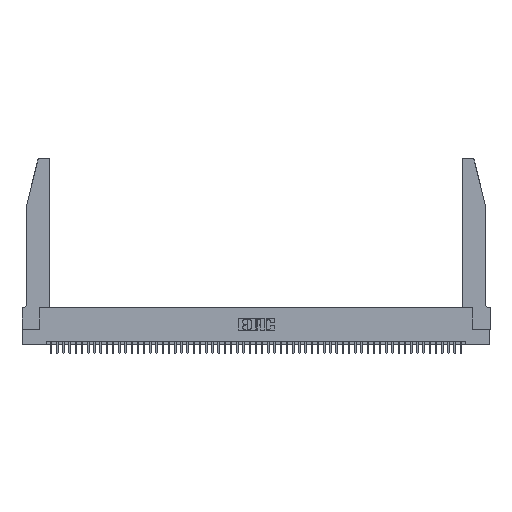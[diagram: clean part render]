
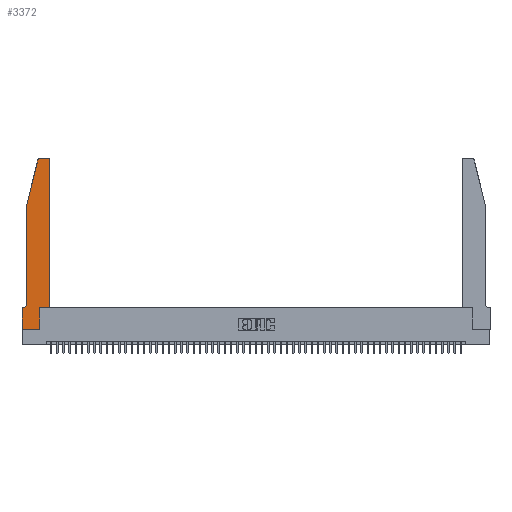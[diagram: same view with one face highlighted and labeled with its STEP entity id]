
A CAD part, top view. The second image highlights one B-rep face of the part: STEP entity #3372.
In plain terms, the highlighted planar face has unit normal (0, 0, 1).
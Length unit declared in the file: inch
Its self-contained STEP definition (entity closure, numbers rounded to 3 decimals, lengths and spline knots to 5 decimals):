
#15 = EDGE_CURVE ( 'NONE', #44403, #13688, #19117, .T. ) ;
#131 = VECTOR ( 'NONE', #29514, 39.37008 ) ;
#475 = ORIENTED_EDGE ( 'NONE', *, *, #31241, .T. ) ;
#2069 = CARTESIAN_POINT ( 'NONE',  ( 0.0755, 2., 0.37 ) ) ;
#2253 = CARTESIAN_POINT ( 'NONE',  ( 0.0755, 0.35, 0.37 ) ) ;
#2636 = CIRCLE ( 'NONE', #48445, 0.03 ) ;
#3372 = ADVANCED_FACE ( 'NONE', ( #43857 ), #22199, .T. ) ;
#3374 = CARTESIAN_POINT ( 'NONE',  ( 0., 0.35, 0.37 ) ) ;
#3427 = VECTOR ( 'NONE', #8795, 39.37008 ) ;
#3840 = LINE ( 'NONE', #7903, #22732 ) ;
#4207 = CARTESIAN_POINT ( 'NONE',  ( 0.284, 2.75, 0.37 ) ) ;
#5001 = CARTESIAN_POINT ( 'NONE',  ( 0.2865, 0.35, 0.37 ) ) ;
#5003 = DIRECTION ( 'NONE',  ( -1., 0., 0. ) ) ;
#5638 = CARTESIAN_POINT ( 'NONE',  ( 0., 0., 0.37 ) ) ;
#6125 = VERTEX_POINT ( 'NONE', #37381 ) ;
#6273 = DIRECTION ( 'NONE',  ( 0., 0., -1. ) ) ;
#7343 = CARTESIAN_POINT ( 'NONE',  ( 0.0055, 0.35, 0.37 ) ) ;
#7903 = CARTESIAN_POINT ( 'NONE',  ( 0., 0., 0.37 ) ) ;
#8156 = LINE ( 'NONE', #51438, #11471 ) ;
#8225 = AXIS2_PLACEMENT_3D ( 'NONE', #10287, #6273, #47514 ) ;
#8795 = DIRECTION ( 'NONE',  ( 0., 1., 0. ) ) ;
#8818 = VECTOR ( 'NONE', #5003, 39.37008 ) ;
#9454 = LINE ( 'NONE', #33608, #8818 ) ;
#9557 = ORIENTED_EDGE ( 'NONE', *, *, #22637, .T. ) ;
#10287 = CARTESIAN_POINT ( 'NONE',  ( 0.0055, 0.42, 0.37 ) ) ;
#10353 = ORIENTED_EDGE ( 'NONE', *, *, #49988, .T. ) ;
#11436 = VERTEX_POINT ( 'NONE', #46766 ) ;
#11471 = VECTOR ( 'NONE', #38810, 39.37008 ) ;
#12121 = CARTESIAN_POINT ( 'NONE',  ( 0.4505, 0.35, 0.37 ) ) ;
#13207 = EDGE_CURVE ( 'NONE', #17893, #53528, #9454, .T. ) ;
#13651 = AXIS2_PLACEMENT_3D ( 'NONE', #33407, #46001, #38130 ) ;
#13688 = VERTEX_POINT ( 'NONE', #25513 ) ;
#13776 = VECTOR ( 'NONE', #32651, 39.37008 ) ;
#14187 = CARTESIAN_POINT ( 'NONE',  ( 0., 0.35, 0.37 ) ) ;
#14417 = LINE ( 'NONE', #33371, #13776 ) ;
#16508 = CARTESIAN_POINT ( 'NONE',  ( 0.2865, 0.35, 0.37 ) ) ;
#17020 = ORIENTED_EDGE ( 'NONE', *, *, #46171, .T. ) ;
#17547 = EDGE_LOOP ( 'NONE', ( #25441, #10353, #23914, #53851, #41635, #17020, #37264, #475, #22354, #9557, #35073, #46876 ) ) ;
#17709 = LINE ( 'NONE', #5001, #3427 ) ;
#17893 = VERTEX_POINT ( 'NONE', #32282 ) ;
#18748 = DIRECTION ( 'NONE',  ( 1., 0., 0. ) ) ;
#18919 = CARTESIAN_POINT ( 'NONE',  ( 0.4505, 0.35, 0.37 ) ) ;
#19117 = LINE ( 'NONE', #49888, #23032 ) ;
#20321 = DIRECTION ( 'NONE',  ( 0., 1., 0. ) ) ;
#22199 = PLANE ( 'NONE',  #30518 ) ;
#22354 = ORIENTED_EDGE ( 'NONE', *, *, #29598, .T. ) ;
#22637 = EDGE_CURVE ( 'NONE', #49591, #53800, #14417, .T. ) ;
#22732 = VECTOR ( 'NONE', #45690, 39.37008 ) ;
#22969 = LINE ( 'NONE', #12121, #39924 ) ;
#23032 = VECTOR ( 'NONE', #45841, 39.37008 ) ;
#23645 = CARTESIAN_POINT ( 'NONE',  ( 0.4505, 2.72, 0.37 ) ) ;
#23914 = ORIENTED_EDGE ( 'NONE', *, *, #40170, .T. ) ;
#25441 = ORIENTED_EDGE ( 'NONE', *, *, #13207, .T. ) ;
#25513 = CARTESIAN_POINT ( 'NONE',  ( 0.0755, 0.42, 0.37 ) ) ;
#26987 = DIRECTION ( 'NONE',  ( -1., 0., 0. ) ) ;
#29514 = DIRECTION ( 'NONE',  ( -0.239, -0.971, 0. ) ) ;
#29598 = EDGE_CURVE ( 'NONE', #6125, #49591, #17709, .T. ) ;
#30518 = AXIS2_PLACEMENT_3D ( 'NONE', #14187, #43357, #18748 ) ;
#31241 = EDGE_CURVE ( 'NONE', #50080, #6125, #3840, .T. ) ;
#32282 = CARTESIAN_POINT ( 'NONE',  ( 0.4205, 2.75, 0.37 ) ) ;
#32651 = DIRECTION ( 'NONE',  ( 1., 0., 0. ) ) ;
#33371 = CARTESIAN_POINT ( 'NONE',  ( 0.4505, 0.35, 0.37 ) ) ;
#33407 = CARTESIAN_POINT ( 'NONE',  ( 0.4205, 2.72, 0.37 ) ) ;
#33608 = CARTESIAN_POINT ( 'NONE',  ( 0.2605, 2.75, 0.37 ) ) ;
#33948 = VERTEX_POINT ( 'NONE', #7343 ) ;
#35073 = ORIENTED_EDGE ( 'NONE', *, *, #45262, .T. ) ;
#37264 = ORIENTED_EDGE ( 'NONE', *, *, #52009, .T. ) ;
#37381 = CARTESIAN_POINT ( 'NONE',  ( 0.2865, 0., 0.37 ) ) ;
#37909 = CARTESIAN_POINT ( 'NONE',  ( 0.0755, 2., 0.37 ) ) ;
#38130 = DIRECTION ( 'NONE',  ( 1., 0., 0. ) ) ;
#38367 = CIRCLE ( 'NONE', #8225, 0.07 ) ;
#38810 = DIRECTION ( 'NONE',  ( 0., -1., 0. ) ) ;
#39444 = CARTESIAN_POINT ( 'NONE',  ( 0.284, 2.72, 0.37 ) ) ;
#39924 = VECTOR ( 'NONE', #20321, 39.37008 ) ;
#40170 = EDGE_CURVE ( 'NONE', #11436, #44403, #51033, .T. ) ;
#40650 = VERTEX_POINT ( 'NONE', #23645 ) ;
#41635 = ORIENTED_EDGE ( 'NONE', *, *, #50656, .T. ) ;
#42453 = VECTOR ( 'NONE', #26987, 39.37008 ) ;
#42697 = VERTEX_POINT ( 'NONE', #3374 ) ;
#43357 = DIRECTION ( 'NONE',  ( 0., 0., 1. ) ) ;
#43652 = DIRECTION ( 'NONE',  ( 0., 0., 1. ) ) ;
#43857 = FACE_OUTER_BOUND ( 'NONE', #17547, .T. ) ;
#44403 = VERTEX_POINT ( 'NONE', #2069 ) ;
#45262 = EDGE_CURVE ( 'NONE', #53800, #40650, #22969, .T. ) ;
#45690 = DIRECTION ( 'NONE',  ( 1., 0., 0. ) ) ;
#45841 = DIRECTION ( 'NONE',  ( 0., -1., 0. ) ) ;
#45859 = EDGE_CURVE ( 'NONE', #40650, #17893, #51003, .T. ) ;
#46001 = DIRECTION ( 'NONE',  ( 0., 0., 1. ) ) ;
#46171 = EDGE_CURVE ( 'NONE', #33948, #42697, #47013, .T. ) ;
#46766 = CARTESIAN_POINT ( 'NONE',  ( 0.25487, 2.72718, 0.37 ) ) ;
#46876 = ORIENTED_EDGE ( 'NONE', *, *, #45859, .T. ) ;
#47013 = LINE ( 'NONE', #2253, #42453 ) ;
#47514 = DIRECTION ( 'NONE',  ( -1., 0., 0. ) ) ;
#47848 = DIRECTION ( 'NONE',  ( 1., 0., 0. ) ) ;
#48445 = AXIS2_PLACEMENT_3D ( 'NONE', #39444, #43652, #47848 ) ;
#49591 = VERTEX_POINT ( 'NONE', #16508 ) ;
#49888 = CARTESIAN_POINT ( 'NONE',  ( 0.0755, 2., 0.37 ) ) ;
#49988 = EDGE_CURVE ( 'NONE', #53528, #11436, #2636, .T. ) ;
#50080 = VERTEX_POINT ( 'NONE', #5638 ) ;
#50656 = EDGE_CURVE ( 'NONE', #13688, #33948, #38367, .T. ) ;
#51003 = CIRCLE ( 'NONE', #13651, 0.03 ) ;
#51033 = LINE ( 'NONE', #37909, #131 ) ;
#51438 = CARTESIAN_POINT ( 'NONE',  ( 0., 0., 0.37 ) ) ;
#52009 = EDGE_CURVE ( 'NONE', #42697, #50080, #8156, .T. ) ;
#53528 = VERTEX_POINT ( 'NONE', #4207 ) ;
#53800 = VERTEX_POINT ( 'NONE', #18919 ) ;
#53851 = ORIENTED_EDGE ( 'NONE', *, *, #15, .T. ) ;
